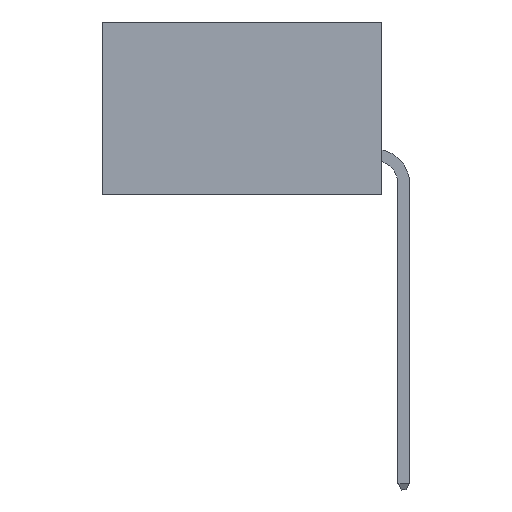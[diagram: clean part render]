
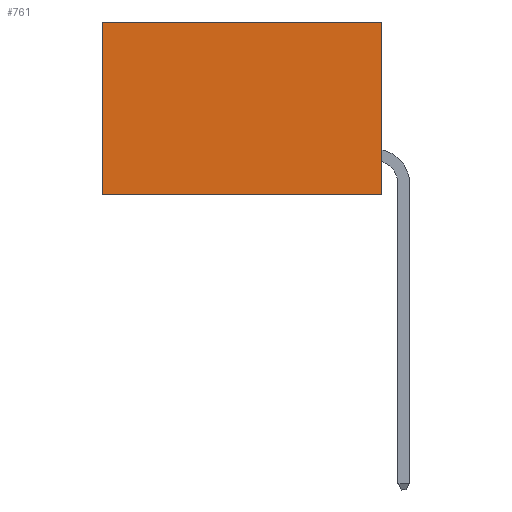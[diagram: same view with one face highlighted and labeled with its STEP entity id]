
A CAD part, left-side view. The second image highlights one B-rep face of the part: STEP entity #761.
In plain terms, the highlighted planar face has unit normal (-1, 0, 0).
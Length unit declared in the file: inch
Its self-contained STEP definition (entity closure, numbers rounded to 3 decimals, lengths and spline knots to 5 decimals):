
#50 = CARTESIAN_POINT ( 'NONE',  ( 0.2875, 0., 0. ) ) ;
#696 = VERTEX_POINT ( 'NONE', #27487 ) ;
#761 = ADVANCED_FACE ( 'NONE', ( #28476 ), #27629, .F. ) ;
#984 = VERTEX_POINT ( 'NONE', #10634 ) ;
#1266 = EDGE_CURVE ( 'NONE', #26764, #696, #27071, .T. ) ;
#1736 = CARTESIAN_POINT ( 'NONE',  ( 0.2875, 0.6, 0. ) ) ;
#1865 = CARTESIAN_POINT ( 'NONE',  ( 0.2875, 0., 0. ) ) ;
#2539 = CARTESIAN_POINT ( 'NONE',  ( 0.2875, 0.6, 0. ) ) ;
#2651 = LINE ( 'NONE', #9726, #26429 ) ;
#3206 = VECTOR ( 'NONE', #3999, 39.37008 ) ;
#3999 = DIRECTION ( 'NONE',  ( 0., 0., -1. ) ) ;
#5086 = CARTESIAN_POINT ( 'NONE',  ( 0.2875, 0., 0. ) ) ;
#7275 = DIRECTION ( 'NONE',  ( 1., 0., 0. ) ) ;
#8799 = EDGE_CURVE ( 'NONE', #696, #984, #2651, .T. ) ;
#9726 = CARTESIAN_POINT ( 'NONE',  ( 0.2875, 0., -0.37 ) ) ;
#10492 = EDGE_LOOP ( 'NONE', ( #17137, #28748, #14234, #27643 ) ) ;
#10634 = CARTESIAN_POINT ( 'NONE',  ( 0.2875, 0.6, -0.37 ) ) ;
#11873 = VERTEX_POINT ( 'NONE', #2539 ) ;
#11992 = DIRECTION ( 'NONE',  ( 0., 1., 0. ) ) ;
#14234 = ORIENTED_EDGE ( 'NONE', *, *, #1266, .F. ) ;
#15156 = LINE ( 'NONE', #1736, #3206 ) ;
#15495 = AXIS2_PLACEMENT_3D ( 'NONE', #1865, #7275, #26520 ) ;
#15588 = EDGE_CURVE ( 'NONE', #11873, #984, #15156, .T. ) ;
#17137 = ORIENTED_EDGE ( 'NONE', *, *, #15588, .T. ) ;
#18007 = DIRECTION ( 'NONE',  ( 0., 1., 0. ) ) ;
#19624 = LINE ( 'NONE', #50, #24840 ) ;
#20542 = EDGE_CURVE ( 'NONE', #26764, #11873, #19624, .T. ) ;
#21902 = VECTOR ( 'NONE', #26481, 39.37008 ) ;
#24796 = CARTESIAN_POINT ( 'NONE',  ( 0.2875, 0., 0. ) ) ;
#24840 = VECTOR ( 'NONE', #18007, 39.37008 ) ;
#26429 = VECTOR ( 'NONE', #11992, 39.37008 ) ;
#26481 = DIRECTION ( 'NONE',  ( 0., 0., -1. ) ) ;
#26520 = DIRECTION ( 'NONE',  ( 0., 0., -1. ) ) ;
#26764 = VERTEX_POINT ( 'NONE', #24796 ) ;
#27071 = LINE ( 'NONE', #5086, #21902 ) ;
#27487 = CARTESIAN_POINT ( 'NONE',  ( 0.2875, 0., -0.37 ) ) ;
#27629 = PLANE ( 'NONE',  #15495 ) ;
#27643 = ORIENTED_EDGE ( 'NONE', *, *, #20542, .T. ) ;
#28476 = FACE_OUTER_BOUND ( 'NONE', #10492, .T. ) ;
#28748 = ORIENTED_EDGE ( 'NONE', *, *, #8799, .F. ) ;
